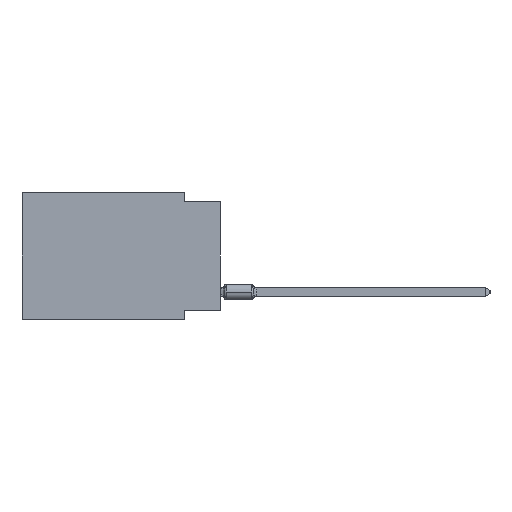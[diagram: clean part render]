
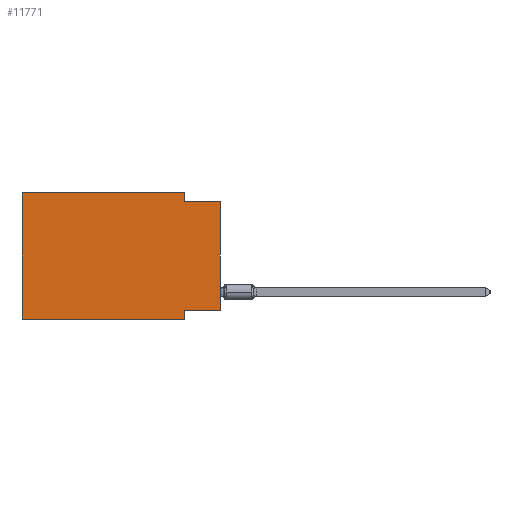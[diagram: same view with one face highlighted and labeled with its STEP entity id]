
A CAD part, left-side view. The second image highlights one B-rep face of the part: STEP entity #11771.
In plain terms, the highlighted planar face has unit normal (-1, 0, 0).
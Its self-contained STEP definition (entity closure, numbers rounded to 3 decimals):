
#268 = FACE_OUTER_BOUND ( 'NONE', #4612, .T. ) ;
#459 = CARTESIAN_POINT ( 'NONE',  ( 0., 13.97, 0. ) ) ;
#915 = EDGE_CURVE ( 'NONE', #2873, #9598, #10159, .T. ) ;
#1194 = VECTOR ( 'NONE', #8514, 1000. ) ;
#1794 = ORIENTED_EDGE ( 'NONE', *, *, #7271, .F. ) ;
#2142 = DIRECTION ( 'NONE',  ( 0., 0., -1. ) ) ;
#2208 = VERTEX_POINT ( 'NONE', #8454 ) ;
#2873 = VERTEX_POINT ( 'NONE', #6058 ) ;
#3009 = VECTOR ( 'NONE', #7658, 1000. ) ;
#3183 = CARTESIAN_POINT ( 'NONE',  ( 0., 13.97, 0. ) ) ;
#3452 = CARTESIAN_POINT ( 'NONE',  ( 0., 0., -0.635 ) ) ;
#3471 = VECTOR ( 'NONE', #13182, 1000. ) ;
#3475 = LINE ( 'NONE', #12060, #8455 ) ;
#3850 = DIRECTION ( 'NONE',  ( 0., 1., 0. ) ) ;
#4343 = ORIENTED_EDGE ( 'NONE', *, *, #6117, .F. ) ;
#4420 = CARTESIAN_POINT ( 'NONE',  ( 0., 0., 0. ) ) ;
#4612 = EDGE_LOOP ( 'NONE', ( #16139, #4343, #17161, #6120, #1794, #7443, #15317, #10152 ) ) ;
#5489 = DIRECTION ( 'NONE',  ( 1., 0., 0. ) ) ;
#5741 = EDGE_CURVE ( 'NONE', #13052, #9598, #17130, .T. ) ;
#6058 = CARTESIAN_POINT ( 'NONE',  ( 0., 13.97, -8.89 ) ) ;
#6117 = EDGE_CURVE ( 'NONE', #16551, #8168, #15547, .T. ) ;
#6120 = ORIENTED_EDGE ( 'NONE', *, *, #11857, .F. ) ;
#6261 = VECTOR ( 'NONE', #3850, 1000. ) ;
#6750 = EDGE_CURVE ( 'NONE', #9366, #16551, #9267, .T. ) ;
#7106 = CARTESIAN_POINT ( 'NONE',  ( 0., 2.54, 0. ) ) ;
#7271 = EDGE_CURVE ( 'NONE', #2873, #9525, #3475, .T. ) ;
#7443 = ORIENTED_EDGE ( 'NONE', *, *, #915, .T. ) ;
#7583 = CARTESIAN_POINT ( 'NONE',  ( 0., 2.54, -8.89 ) ) ;
#7658 = DIRECTION ( 'NONE',  ( 0., -1., 0. ) ) ;
#8168 = VERTEX_POINT ( 'NONE', #3452 ) ;
#8315 = CARTESIAN_POINT ( 'NONE',  ( 0., 13.97, 0. ) ) ;
#8454 = CARTESIAN_POINT ( 'NONE',  ( 0., 0., -8.255 ) ) ;
#8455 = VECTOR ( 'NONE', #16098, 1000. ) ;
#8514 = DIRECTION ( 'NONE',  ( 0., 0., 1. ) ) ;
#8606 = CARTESIAN_POINT ( 'NONE',  ( 0., 13.97, -8.89 ) ) ;
#9267 = LINE ( 'NONE', #16232, #14007 ) ;
#9366 = VERTEX_POINT ( 'NONE', #7106 ) ;
#9525 = VERTEX_POINT ( 'NONE', #3183 ) ;
#9598 = VERTEX_POINT ( 'NONE', #17183 ) ;
#9691 = PLANE ( 'NONE',  #15871 ) ;
#9783 = DIRECTION ( 'NONE',  ( 0., 0., -1. ) ) ;
#10152 = ORIENTED_EDGE ( 'NONE', *, *, #17547, .F. ) ;
#10159 = LINE ( 'NONE', #8606, #14453 ) ;
#10882 = LINE ( 'NONE', #13442, #6261 ) ;
#11525 = CARTESIAN_POINT ( 'NONE',  ( 0., 2.54, -8.255 ) ) ;
#11602 = DIRECTION ( 'NONE',  ( 0., -1., 0. ) ) ;
#11771 = ADVANCED_FACE ( 'NONE', ( #268 ), #9691, .F. ) ;
#11857 = EDGE_CURVE ( 'NONE', #9525, #9366, #17286, .T. ) ;
#12060 = CARTESIAN_POINT ( 'NONE',  ( 0., 13.97, 0. ) ) ;
#12826 = DIRECTION ( 'NONE',  ( 0., -1., 0. ) ) ;
#13052 = VERTEX_POINT ( 'NONE', #11525 ) ;
#13182 = DIRECTION ( 'NONE',  ( 0., 0., -1. ) ) ;
#13442 = CARTESIAN_POINT ( 'NONE',  ( 0., 0., -8.255 ) ) ;
#14007 = VECTOR ( 'NONE', #2142, 1000. ) ;
#14171 = CARTESIAN_POINT ( 'NONE',  ( 0., 0., -0.635 ) ) ;
#14453 = VECTOR ( 'NONE', #12826, 1000. ) ;
#14761 = EDGE_CURVE ( 'NONE', #2208, #8168, #15479, .T. ) ;
#14865 = VECTOR ( 'NONE', #11602, 1000. ) ;
#15105 = CARTESIAN_POINT ( 'NONE',  ( 0., 2.54, -0.635 ) ) ;
#15317 = ORIENTED_EDGE ( 'NONE', *, *, #5741, .F. ) ;
#15479 = LINE ( 'NONE', #4420, #1194 ) ;
#15547 = LINE ( 'NONE', #14171, #14865 ) ;
#15871 = AXIS2_PLACEMENT_3D ( 'NONE', #8315, #5489, #9783 ) ;
#16098 = DIRECTION ( 'NONE',  ( 0., 0., 1. ) ) ;
#16139 = ORIENTED_EDGE ( 'NONE', *, *, #14761, .T. ) ;
#16232 = CARTESIAN_POINT ( 'NONE',  ( 0., 2.54, 0. ) ) ;
#16551 = VERTEX_POINT ( 'NONE', #15105 ) ;
#17130 = LINE ( 'NONE', #7583, #3471 ) ;
#17161 = ORIENTED_EDGE ( 'NONE', *, *, #6750, .F. ) ;
#17183 = CARTESIAN_POINT ( 'NONE',  ( 0., 2.54, -8.89 ) ) ;
#17286 = LINE ( 'NONE', #459, #3009 ) ;
#17547 = EDGE_CURVE ( 'NONE', #2208, #13052, #10882, .T. ) ;
